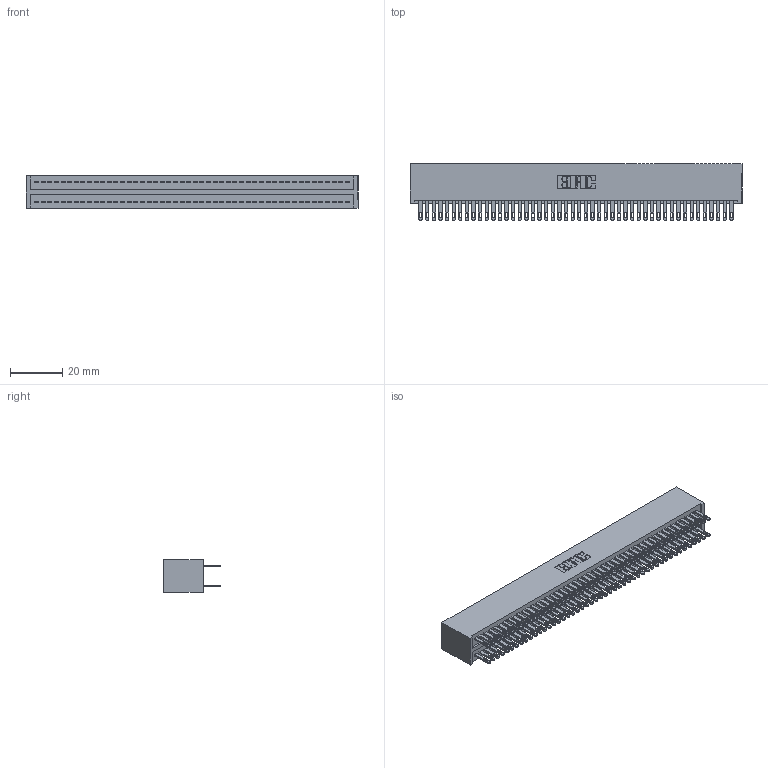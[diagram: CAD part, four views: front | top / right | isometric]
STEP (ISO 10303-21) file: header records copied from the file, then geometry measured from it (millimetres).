
FILE_DESCRIPTION (( 'STEP AP203' ), '1' );
FILE_NAME ('325-096-500-201.STEP', '2020-02-25T06:08:22', ( '' ), ( '' ), 'SwSTEP 2.0', 'SolidWorks 2016', '' );
FILE_SCHEMA (( 'CONFIG_CONTROL_DESIGN' ));
Length unit declared in the file: inch
Products named in the file (3): 325-292-001_325-293-100; 325-096-500-201; 325 Part_Lugless
Assembly tree (97 placements, depth 2):
  325-096-500-201
    325 Part_Lugless
    325-292-001_325-293-100  x96
Bounding box: 127.56 x 21.84 x 12.45 mm (x, y, z)
Volume: 17420.7 mm3; surface area: 22892.5 mm2
Topology: 97 solids, 97 shells, 4714 faces, 14399 edges, 9598 vertices
Faces by surface type: plane 2946, cylinder 1768
Entity records: 29757 total; most frequent: CARTESIAN_POINT 4922, ORIENTED_EDGE 4858, DIRECTION 4189, EDGE_CURVE 2429, VECTOR 2305, LINE 2305, VERTEX_POINT 1618, AXIS2_PLACEMENT_3D 942
